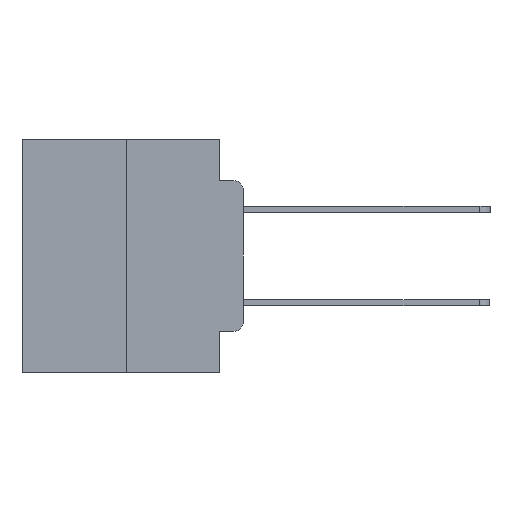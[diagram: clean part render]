
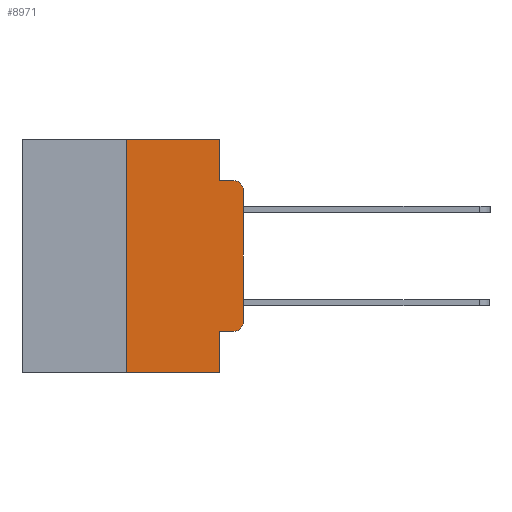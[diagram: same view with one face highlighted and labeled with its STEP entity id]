
A CAD part, left-side view. The second image highlights one B-rep face of the part: STEP entity #8971.
In plain terms, the highlighted planar face has unit normal (-1, 0, 0).
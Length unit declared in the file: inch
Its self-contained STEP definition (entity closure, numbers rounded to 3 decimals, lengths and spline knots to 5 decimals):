
#186 = VERTEX_POINT ( 'NONE', #8590 ) ;
#734 = DIRECTION ( 'NONE',  ( 0., 0., -1. ) ) ;
#825 = EDGE_CURVE ( 'NONE', #1195, #24086, #25750, .T. ) ;
#900 = EDGE_LOOP ( 'NONE', ( #8787, #13498, #21565, #25528, #13520, #1672, #12221, #10969, #10336, #24956 ) ) ;
#1085 = DIRECTION ( 'NONE',  ( 0., -1., 0. ) ) ;
#1195 = VERTEX_POINT ( 'NONE', #4607 ) ;
#1480 = DIRECTION ( 'NONE',  ( 0., 0., 1. ) ) ;
#1672 = ORIENTED_EDGE ( 'NONE', *, *, #2620, .F. ) ;
#1820 = VERTEX_POINT ( 'NONE', #17768 ) ;
#1930 = DIRECTION ( 'NONE',  ( -1., 0., 0. ) ) ;
#2098 = EDGE_CURVE ( 'NONE', #186, #11507, #18856, .T. ) ;
#2504 = VERTEX_POINT ( 'NONE', #4581 ) ;
#2525 = EDGE_CURVE ( 'NONE', #15712, #10400, #14481, .T. ) ;
#2533 = EDGE_CURVE ( 'NONE', #10400, #1820, #24369, .T. ) ;
#2570 = EDGE_CURVE ( 'NONE', #2504, #1820, #13857, .T. ) ;
#2580 = EDGE_CURVE ( 'NONE', #24086, #2504, #9742, .T. ) ;
#2620 = EDGE_CURVE ( 'NONE', #186, #1195, #11275, .T. ) ;
#2631 = EDGE_CURVE ( 'NONE', #18210, #11507, #26485, .T. ) ;
#2666 = EDGE_CURVE ( 'NONE', #18210, #25741, #10680, .T. ) ;
#2671 = EDGE_CURVE ( 'NONE', #25741, #15712, #25268, .T. ) ;
#3587 = VECTOR ( 'NONE', #17244, 39.37008 ) ;
#4066 = CARTESIAN_POINT ( 'NONE',  ( 0., 0.051, -0.4115 ) ) ;
#4581 = CARTESIAN_POINT ( 'NONE',  ( 0., 0.051, -0.0885 ) ) ;
#4607 = CARTESIAN_POINT ( 'NONE',  ( 0., 0.25, 0. ) ) ;
#5260 = VECTOR ( 'NONE', #734, 39.37008 ) ;
#5362 = CARTESIAN_POINT ( 'NONE',  ( 0., 0.02, -0.4115 ) ) ;
#5780 = CARTESIAN_POINT ( 'NONE',  ( 0., 0.02, -0.3915 ) ) ;
#5923 = VECTOR ( 'NONE', #1480, 39.37008 ) ;
#7943 = CARTESIAN_POINT ( 'NONE',  ( 0., 0.051, -0.4115 ) ) ;
#8214 = DIRECTION ( 'NONE',  ( 0., -1., 0. ) ) ;
#8231 = VECTOR ( 'NONE', #1085, 39.37008 ) ;
#8590 = CARTESIAN_POINT ( 'NONE',  ( 0., 0.25, -0.5 ) ) ;
#8787 = ORIENTED_EDGE ( 'NONE', *, *, #2525, .T. ) ;
#8880 = DIRECTION ( 'NONE',  ( 0., 0., -1. ) ) ;
#8971 = ADVANCED_FACE ( 'NONE', ( #11290 ), #20731, .F. ) ;
#9397 = AXIS2_PLACEMENT_3D ( 'NONE', #5780, #19204, #8880 ) ;
#9742 = LINE ( 'NONE', #26144, #22516 ) ;
#9925 = VECTOR ( 'NONE', #17192, 39.37008 ) ;
#10336 = ORIENTED_EDGE ( 'NONE', *, *, #2666, .T. ) ;
#10400 = VERTEX_POINT ( 'NONE', #23064 ) ;
#10680 = LINE ( 'NONE', #7943, #20670 ) ;
#10779 = DIRECTION ( 'NONE',  ( 1., 0., 0. ) ) ;
#10872 = CARTESIAN_POINT ( 'NONE',  ( 0., 0.473, -0.5 ) ) ;
#10969 = ORIENTED_EDGE ( 'NONE', *, *, #2631, .F. ) ;
#11275 = LINE ( 'NONE', #16127, #5923 ) ;
#11290 = FACE_OUTER_BOUND ( 'NONE', #900, .T. ) ;
#11486 = DIRECTION ( 'NONE',  ( 0., 0., -1. ) ) ;
#11507 = VERTEX_POINT ( 'NONE', #16742 ) ;
#12221 = ORIENTED_EDGE ( 'NONE', *, *, #2098, .T. ) ;
#13498 = ORIENTED_EDGE ( 'NONE', *, *, #2533, .T. ) ;
#13520 = ORIENTED_EDGE ( 'NONE', *, *, #825, .F. ) ;
#13857 = LINE ( 'NONE', #14717, #23129 ) ;
#14481 = LINE ( 'NONE', #24176, #3587 ) ;
#14580 = CARTESIAN_POINT ( 'NONE',  ( 0., 0.051, 0. ) ) ;
#14717 = CARTESIAN_POINT ( 'NONE',  ( 0., 0.051, -0.0885 ) ) ;
#15712 = VERTEX_POINT ( 'NONE', #25727 ) ;
#16127 = CARTESIAN_POINT ( 'NONE',  ( 0., 0.25, 0. ) ) ;
#16637 = CARTESIAN_POINT ( 'NONE',  ( 0., 0.02, -0.1085 ) ) ;
#16742 = CARTESIAN_POINT ( 'NONE',  ( 0., 0.051, -0.5 ) ) ;
#17192 = DIRECTION ( 'NONE',  ( 0., -1., 0. ) ) ;
#17244 = DIRECTION ( 'NONE',  ( 0., 0., 1. ) ) ;
#17268 = DIRECTION ( 'NONE',  ( 0., 0., -1. ) ) ;
#17768 = CARTESIAN_POINT ( 'NONE',  ( 0., 0.02, -0.0885 ) ) ;
#18210 = VERTEX_POINT ( 'NONE', #4066 ) ;
#18856 = LINE ( 'NONE', #10872, #8231 ) ;
#19204 = DIRECTION ( 'NONE',  ( -1., 0., 0. ) ) ;
#19791 = CARTESIAN_POINT ( 'NONE',  ( 0., 0.051, 0. ) ) ;
#20670 = VECTOR ( 'NONE', #25903, 39.37008 ) ;
#20731 = PLANE ( 'NONE',  #24297 ) ;
#21565 = ORIENTED_EDGE ( 'NONE', *, *, #2570, .F. ) ;
#22516 = VECTOR ( 'NONE', #17268, 39.37008 ) ;
#23064 = CARTESIAN_POINT ( 'NONE',  ( 0., 0., -0.1085 ) ) ;
#23129 = VECTOR ( 'NONE', #8214, 39.37008 ) ;
#23228 = AXIS2_PLACEMENT_3D ( 'NONE', #16637, #1930, #11486 ) ;
#23350 = CARTESIAN_POINT ( 'NONE',  ( 0., 0.473, 0. ) ) ;
#24086 = VERTEX_POINT ( 'NONE', #14580 ) ;
#24176 = CARTESIAN_POINT ( 'NONE',  ( 0., 0., 0. ) ) ;
#24297 = AXIS2_PLACEMENT_3D ( 'NONE', #24508, #10779, #24686 ) ;
#24369 = CIRCLE ( 'NONE', #23228, 0.02 ) ;
#24508 = CARTESIAN_POINT ( 'NONE',  ( 0., 0.473, 0. ) ) ;
#24686 = DIRECTION ( 'NONE',  ( 0., 0., -1. ) ) ;
#24956 = ORIENTED_EDGE ( 'NONE', *, *, #2671, .T. ) ;
#25268 = CIRCLE ( 'NONE', #9397, 0.02 ) ;
#25528 = ORIENTED_EDGE ( 'NONE', *, *, #2580, .F. ) ;
#25727 = CARTESIAN_POINT ( 'NONE',  ( 0., 0., -0.3915 ) ) ;
#25741 = VERTEX_POINT ( 'NONE', #5362 ) ;
#25750 = LINE ( 'NONE', #23350, #9925 ) ;
#25903 = DIRECTION ( 'NONE',  ( 0., -1., 0. ) ) ;
#26144 = CARTESIAN_POINT ( 'NONE',  ( 0., 0.051, 0. ) ) ;
#26485 = LINE ( 'NONE', #19791, #5260 ) ;
